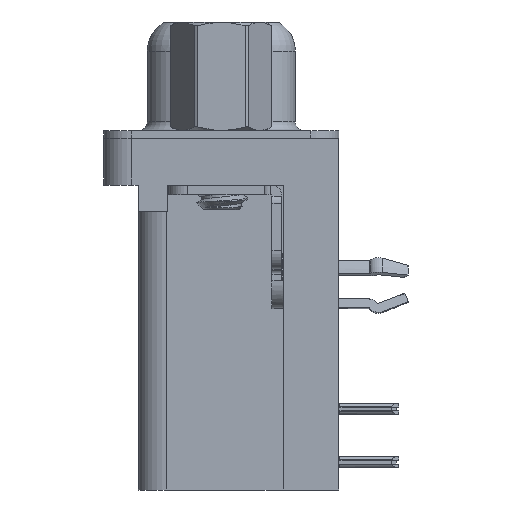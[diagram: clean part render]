
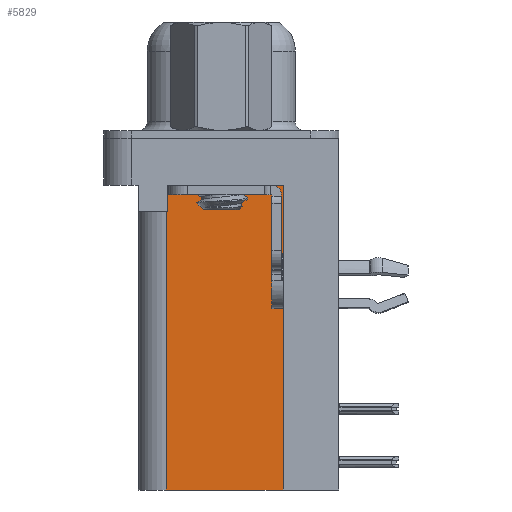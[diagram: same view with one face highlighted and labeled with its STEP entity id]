
A CAD part, left-side view. The second image highlights one B-rep face of the part: STEP entity #5829.
In plain terms, the highlighted planar face has unit normal (-1, 0, 0).
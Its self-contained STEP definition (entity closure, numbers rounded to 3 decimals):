
#1427 = CARTESIAN_POINT ( 'NONE',  ( 3.7, -3.295, -18.76 ) ) ;
#1909 = VERTEX_POINT ( 'NONE', #23147 ) ;
#2658 = ORIENTED_EDGE ( 'NONE', *, *, #19013, .T. ) ;
#2930 = ORIENTED_EDGE ( 'NONE', *, *, #4984, .F. ) ;
#3349 = EDGE_CURVE ( 'NONE', #5375, #25482, #28398, .T. ) ;
#3594 = VECTOR ( 'NONE', #24486, 1000. ) ;
#3716 = LINE ( 'NONE', #24608, #3594 ) ;
#4039 = DIRECTION ( 'NONE',  ( 0., 1., 0. ) ) ;
#4984 = EDGE_CURVE ( 'NONE', #21184, #5375, #13639, .T. ) ;
#5375 = VERTEX_POINT ( 'NONE', #26669 ) ;
#5599 = EDGE_CURVE ( 'NONE', #21184, #1909, #9878, .T. ) ;
#5829 = ADVANCED_FACE ( 'NONE', ( #8279 ), #33327, .F. ) ;
#6092 = DIRECTION ( 'NONE',  ( 0., 1., 0. ) ) ;
#6903 = VERTEX_POINT ( 'NONE', #14609 ) ;
#7008 = ORIENTED_EDGE ( 'NONE', *, *, #10328, .T. ) ;
#8279 = FACE_OUTER_BOUND ( 'NONE', #30918, .T. ) ;
#9359 = ORIENTED_EDGE ( 'NONE', *, *, #5599, .T. ) ;
#9878 = LINE ( 'NONE', #11304, #9980 ) ;
#9980 = VECTOR ( 'NONE', #32405, 1000. ) ;
#10174 = VECTOR ( 'NONE', #18003, 1000. ) ;
#10265 = LINE ( 'NONE', #33638, #10174 ) ;
#10328 = EDGE_CURVE ( 'NONE', #6903, #25482, #13880, .T. ) ;
#11304 = CARTESIAN_POINT ( 'NONE',  ( 3.7, -3.295, -18.76 ) ) ;
#12000 = ORIENTED_EDGE ( 'NONE', *, *, #17653, .T. ) ;
#12787 = CARTESIAN_POINT ( 'NONE',  ( 3.7, 2.895, -2.5 ) ) ;
#13084 = CARTESIAN_POINT ( 'NONE',  ( 3.7, -3.295, -18.76 ) ) ;
#13639 = LINE ( 'NONE', #30252, #13822 ) ;
#13692 = DIRECTION ( 'NONE',  ( 0., 0., 1. ) ) ;
#13708 = VECTOR ( 'NONE', #21767, 1000. ) ;
#13774 = CARTESIAN_POINT ( 'NONE',  ( 3.7, 2.925, -18.76 ) ) ;
#13822 = VECTOR ( 'NONE', #6092, 1000. ) ;
#13880 = LINE ( 'NONE', #19147, #13708 ) ;
#14609 = CARTESIAN_POINT ( 'NONE',  ( 3.7, 2.895, -3.9 ) ) ;
#17653 = EDGE_CURVE ( 'NONE', #1909, #32132, #10265, .T. ) ;
#18003 = DIRECTION ( 'NONE',  ( 0., 1., 0. ) ) ;
#19013 = EDGE_CURVE ( 'NONE', #32132, #6903, #3716, .T. ) ;
#19147 = CARTESIAN_POINT ( 'NONE',  ( 3.7, 0., -3.9 ) ) ;
#20331 = DIRECTION ( 'NONE',  ( 1., 0., 0. ) ) ;
#21184 = VERTEX_POINT ( 'NONE', #13084 ) ;
#21551 = CARTESIAN_POINT ( 'NONE',  ( 3.7, 2.925, -3.9 ) ) ;
#21767 = DIRECTION ( 'NONE',  ( 0., 1., 0. ) ) ;
#23147 = CARTESIAN_POINT ( 'NONE',  ( 3.7, -3.295, -2.5 ) ) ;
#24486 = DIRECTION ( 'NONE',  ( 0., 0., -1. ) ) ;
#24608 = CARTESIAN_POINT ( 'NONE',  ( 3.7, 2.895, -3.9 ) ) ;
#25482 = VERTEX_POINT ( 'NONE', #21551 ) ;
#26669 = CARTESIAN_POINT ( 'NONE',  ( 3.7, 2.925, -18.76 ) ) ;
#28176 = VECTOR ( 'NONE', #13692, 1000. ) ;
#28398 = LINE ( 'NONE', #13774, #28176 ) ;
#29960 = AXIS2_PLACEMENT_3D ( 'NONE', #1427, #20331, #4039 ) ;
#30252 = CARTESIAN_POINT ( 'NONE',  ( 3.7, -3.295, -18.76 ) ) ;
#30918 = EDGE_LOOP ( 'NONE', ( #12000, #2658, #7008, #31396, #2930, #9359 ) ) ;
#31396 = ORIENTED_EDGE ( 'NONE', *, *, #3349, .F. ) ;
#32132 = VERTEX_POINT ( 'NONE', #12787 ) ;
#32405 = DIRECTION ( 'NONE',  ( 0., 0., 1. ) ) ;
#33327 = PLANE ( 'NONE',  #29960 ) ;
#33638 = CARTESIAN_POINT ( 'NONE',  ( 3.7, -3.295, -2.5 ) ) ;
